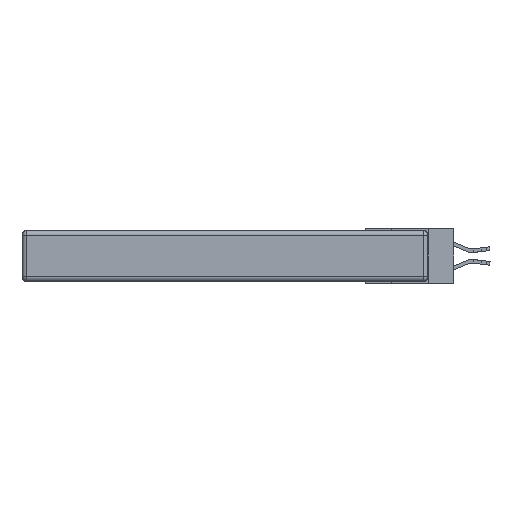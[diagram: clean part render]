
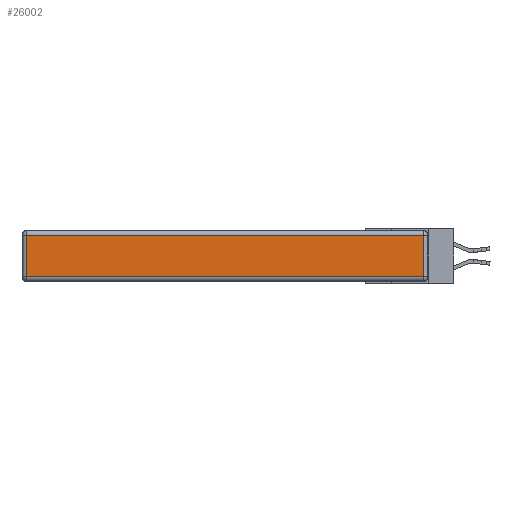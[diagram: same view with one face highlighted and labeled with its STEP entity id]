
A CAD part, left-side view. The second image highlights one B-rep face of the part: STEP entity #26002.
In plain terms, the highlighted planar face has unit normal (-1, 0, 0).
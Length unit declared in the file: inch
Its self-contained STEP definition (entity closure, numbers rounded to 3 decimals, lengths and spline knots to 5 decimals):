
#344 = DIRECTION ( 'NONE',  ( 0., 0., -1. ) ) ;
#914 = LINE ( 'NONE', #19717, #20884 ) ;
#2883 = EDGE_CURVE ( 'NONE', #15387, #10359, #8810, .T. ) ;
#3503 = ORIENTED_EDGE ( 'NONE', *, *, #5852, .T. ) ;
#3919 = VECTOR ( 'NONE', #4665, 39.37008 ) ;
#3937 = CARTESIAN_POINT ( 'NONE',  ( 0., 2.72, -0.313 ) ) ;
#4665 = DIRECTION ( 'NONE',  ( 0., 1., 0. ) ) ;
#5852 = EDGE_CURVE ( 'NONE', #10359, #21521, #12494, .T. ) ;
#6028 = VECTOR ( 'NONE', #20200, 39.37008 ) ;
#6189 = EDGE_LOOP ( 'NONE', ( #22043, #3503, #26287, #27587 ) ) ;
#8174 = AXIS2_PLACEMENT_3D ( 'NONE', #19989, #24071, #9017 ) ;
#8810 = LINE ( 'NONE', #12054, #20674 ) ;
#9017 = DIRECTION ( 'NONE',  ( 0., 0., 1. ) ) ;
#10359 = VERTEX_POINT ( 'NONE', #18535 ) ;
#11586 = EDGE_CURVE ( 'NONE', #21521, #19085, #22539, .T. ) ;
#12054 = CARTESIAN_POINT ( 'NONE',  ( 0., 0., -0.313 ) ) ;
#12494 = LINE ( 'NONE', #19933, #6028 ) ;
#15387 = VERTEX_POINT ( 'NONE', #3937 ) ;
#15468 = CARTESIAN_POINT ( 'NONE',  ( 0., 2.75, -0.03 ) ) ;
#15560 = PLANE ( 'NONE',  #8174 ) ;
#18535 = CARTESIAN_POINT ( 'NONE',  ( 0., 0.03, -0.313 ) ) ;
#18834 = DIRECTION ( 'NONE',  ( 0., -1., 0. ) ) ;
#19085 = VERTEX_POINT ( 'NONE', #22191 ) ;
#19717 = CARTESIAN_POINT ( 'NONE',  ( 0., 2.72, -0.343 ) ) ;
#19933 = CARTESIAN_POINT ( 'NONE',  ( 0., 0.03, -0.343 ) ) ;
#19989 = CARTESIAN_POINT ( 'NONE',  ( 0., 0., -0.343 ) ) ;
#20200 = DIRECTION ( 'NONE',  ( 0., 0., 1. ) ) ;
#20674 = VECTOR ( 'NONE', #18834, 39.37008 ) ;
#20884 = VECTOR ( 'NONE', #344, 39.37008 ) ;
#20940 = FACE_OUTER_BOUND ( 'NONE', #6189, .T. ) ;
#21521 = VERTEX_POINT ( 'NONE', #23388 ) ;
#22043 = ORIENTED_EDGE ( 'NONE', *, *, #2883, .T. ) ;
#22191 = CARTESIAN_POINT ( 'NONE',  ( 0., 2.72, -0.03 ) ) ;
#22539 = LINE ( 'NONE', #15468, #3919 ) ;
#23388 = CARTESIAN_POINT ( 'NONE',  ( 0., 0.03, -0.03 ) ) ;
#24071 = DIRECTION ( 'NONE',  ( -1., 0., 0. ) ) ;
#26002 = ADVANCED_FACE ( 'NONE', ( #20940 ), #15560, .T. ) ;
#26287 = ORIENTED_EDGE ( 'NONE', *, *, #11586, .T. ) ;
#26798 = EDGE_CURVE ( 'NONE', #19085, #15387, #914, .T. ) ;
#27587 = ORIENTED_EDGE ( 'NONE', *, *, #26798, .T. ) ;
